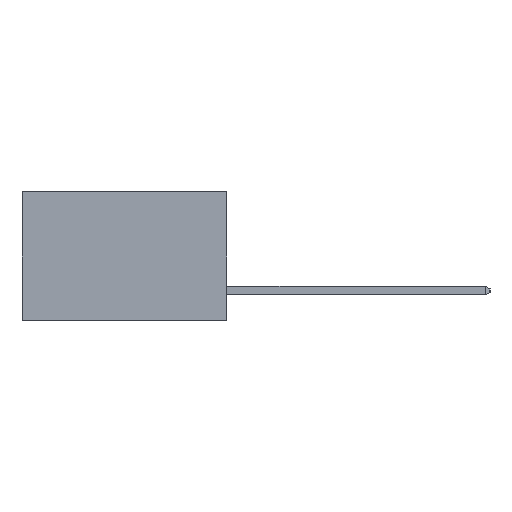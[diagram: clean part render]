
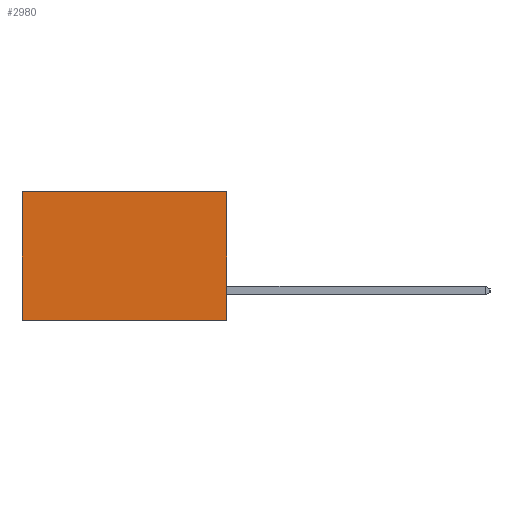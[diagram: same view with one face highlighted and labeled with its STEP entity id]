
A CAD part, left-side view. The second image highlights one B-rep face of the part: STEP entity #2980.
In plain terms, the highlighted planar face has unit normal (-1, 0, 0).
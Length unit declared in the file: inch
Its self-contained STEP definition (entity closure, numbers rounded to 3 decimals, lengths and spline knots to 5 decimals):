
#17 = DIRECTION ( 'NONE',  ( 0., 0., -1. ) ) ;
#236 = DIRECTION ( 'NONE',  ( 1., 0., 0. ) ) ;
#1719 = ORIENTED_EDGE ( 'NONE', *, *, #17180, .F. ) ;
#2165 = VERTEX_POINT ( 'NONE', #2344 ) ;
#2344 = CARTESIAN_POINT ( 'NONE',  ( 0.277, 0.59, 0. ) ) ;
#2980 = ADVANCED_FACE ( 'NONE', ( #19443 ), #13436, .F. ) ;
#3706 = EDGE_LOOP ( 'NONE', ( #6985, #1719, #4294, #5590 ) ) ;
#4294 = ORIENTED_EDGE ( 'NONE', *, *, #14865, .F. ) ;
#4444 = VERTEX_POINT ( 'NONE', #23626 ) ;
#5093 = LINE ( 'NONE', #21721, #19370 ) ;
#5590 = ORIENTED_EDGE ( 'NONE', *, *, #18456, .T. ) ;
#5881 = DIRECTION ( 'NONE',  ( 0., 0., -1. ) ) ;
#6985 = ORIENTED_EDGE ( 'NONE', *, *, #22898, .T. ) ;
#7680 = LINE ( 'NONE', #14737, #19525 ) ;
#8138 = VECTOR ( 'NONE', #16991, 39.37008 ) ;
#8436 = VERTEX_POINT ( 'NONE', #15515 ) ;
#11414 = CARTESIAN_POINT ( 'NONE',  ( 0.277, 0., 0. ) ) ;
#12627 = DIRECTION ( 'NONE',  ( 0., 0., -1. ) ) ;
#12741 = CARTESIAN_POINT ( 'NONE',  ( 0.277, 0., 0. ) ) ;
#12825 = CARTESIAN_POINT ( 'NONE',  ( 0.277, 0., -0.37 ) ) ;
#13436 = PLANE ( 'NONE',  #15419 ) ;
#13718 = LINE ( 'NONE', #11414, #8138 ) ;
#14467 = VECTOR ( 'NONE', #5881, 39.37008 ) ;
#14737 = CARTESIAN_POINT ( 'NONE',  ( 0.277, 0., -0.37 ) ) ;
#14865 = EDGE_CURVE ( 'NONE', #20853, #8436, #5093, .T. ) ;
#15419 = AXIS2_PLACEMENT_3D ( 'NONE', #12825, #236, #17 ) ;
#15515 = CARTESIAN_POINT ( 'NONE',  ( 0.277, 0., -0.37 ) ) ;
#16608 = DIRECTION ( 'NONE',  ( 0., 1., 0. ) ) ;
#16991 = DIRECTION ( 'NONE',  ( 0., 1., 0. ) ) ;
#17061 = CARTESIAN_POINT ( 'NONE',  ( 0.277, 0.59, -0.37 ) ) ;
#17180 = EDGE_CURVE ( 'NONE', #8436, #4444, #7680, .T. ) ;
#18456 = EDGE_CURVE ( 'NONE', #20853, #2165, #13718, .T. ) ;
#19370 = VECTOR ( 'NONE', #12627, 39.37008 ) ;
#19443 = FACE_OUTER_BOUND ( 'NONE', #3706, .T. ) ;
#19525 = VECTOR ( 'NONE', #16608, 39.37008 ) ;
#19871 = LINE ( 'NONE', #17061, #14467 ) ;
#20853 = VERTEX_POINT ( 'NONE', #12741 ) ;
#21721 = CARTESIAN_POINT ( 'NONE',  ( 0.277, 0., -0.37 ) ) ;
#22898 = EDGE_CURVE ( 'NONE', #2165, #4444, #19871, .T. ) ;
#23626 = CARTESIAN_POINT ( 'NONE',  ( 0.277, 0.59, -0.37 ) ) ;
